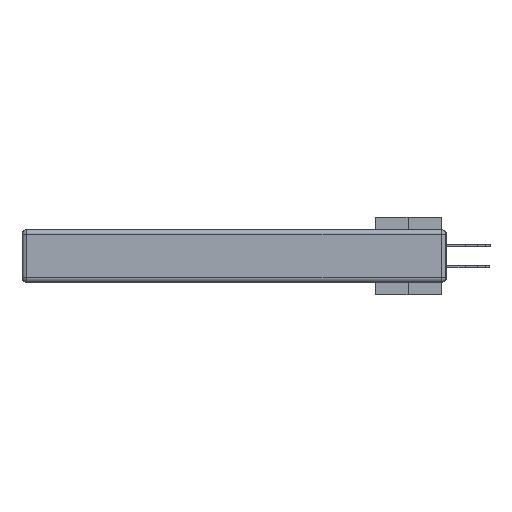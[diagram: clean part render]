
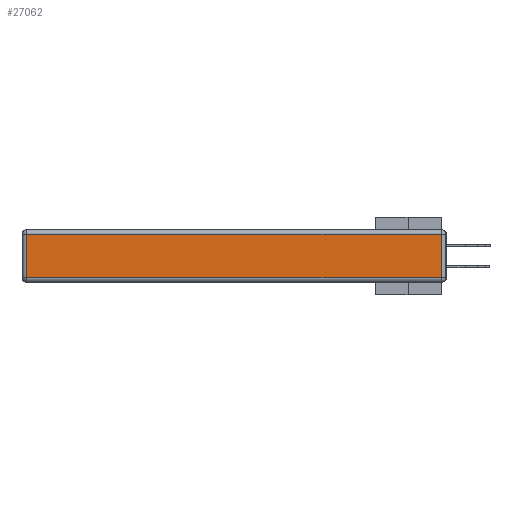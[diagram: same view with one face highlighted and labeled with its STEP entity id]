
A CAD part, left-side view. The second image highlights one B-rep face of the part: STEP entity #27062.
In plain terms, the highlighted planar face has unit normal (-1, 0, 0).
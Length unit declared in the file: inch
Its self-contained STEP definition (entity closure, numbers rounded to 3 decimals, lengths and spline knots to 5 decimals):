
#380 = VERTEX_POINT ( 'NONE', #498 ) ;
#498 = CARTESIAN_POINT ( 'NONE',  ( 0., 0.03, -0.03 ) ) ;
#3220 = VECTOR ( 'NONE', #11821, 39.37008 ) ;
#5016 = CARTESIAN_POINT ( 'NONE',  ( 0., 0., -0.343 ) ) ;
#7217 = VERTEX_POINT ( 'NONE', #21362 ) ;
#7715 = CARTESIAN_POINT ( 'NONE',  ( 0., 0.03, -0.313 ) ) ;
#9782 = VECTOR ( 'NONE', #29040, 39.37008 ) ;
#9840 = ORIENTED_EDGE ( 'NONE', *, *, #22246, .T. ) ;
#11810 = EDGE_CURVE ( 'NONE', #7217, #14208, #23583, .T. ) ;
#11821 = DIRECTION ( 'NONE',  ( 0., 0., 1. ) ) ;
#12468 = EDGE_CURVE ( 'NONE', #20506, #7217, #20412, .T. ) ;
#13033 = CARTESIAN_POINT ( 'NONE',  ( 0., 0., -0.313 ) ) ;
#14208 = VERTEX_POINT ( 'NONE', #7715 ) ;
#14841 = DIRECTION ( 'NONE',  ( 0., 0., 1. ) ) ;
#16550 = LINE ( 'NONE', #27751, #32990 ) ;
#17614 = CARTESIAN_POINT ( 'NONE',  ( 0., 2.72, -0.343 ) ) ;
#17719 = PLANE ( 'NONE',  #21670 ) ;
#17852 = VECTOR ( 'NONE', #21187, 39.37008 ) ;
#18949 = FACE_OUTER_BOUND ( 'NONE', #33417, .T. ) ;
#20294 = ORIENTED_EDGE ( 'NONE', *, *, #11810, .T. ) ;
#20412 = LINE ( 'NONE', #17614, #17852 ) ;
#20506 = VERTEX_POINT ( 'NONE', #30685 ) ;
#21187 = DIRECTION ( 'NONE',  ( 0., 0., -1. ) ) ;
#21362 = CARTESIAN_POINT ( 'NONE',  ( 0., 2.72, -0.313 ) ) ;
#21670 = AXIS2_PLACEMENT_3D ( 'NONE', #5016, #33962, #14841 ) ;
#22246 = EDGE_CURVE ( 'NONE', #14208, #380, #25757, .T. ) ;
#23583 = LINE ( 'NONE', #13033, #9782 ) ;
#25087 = CARTESIAN_POINT ( 'NONE',  ( 0., 0.03, -0.343 ) ) ;
#25757 = LINE ( 'NONE', #25087, #3220 ) ;
#27062 = ADVANCED_FACE ( 'NONE', ( #18949 ), #17719, .T. ) ;
#27751 = CARTESIAN_POINT ( 'NONE',  ( 0., 2.75, -0.03 ) ) ;
#28865 = ORIENTED_EDGE ( 'NONE', *, *, #39782, .T. ) ;
#29040 = DIRECTION ( 'NONE',  ( 0., -1., 0. ) ) ;
#30685 = CARTESIAN_POINT ( 'NONE',  ( 0., 2.72, -0.03 ) ) ;
#32990 = VECTOR ( 'NONE', #34261, 39.37008 ) ;
#33417 = EDGE_LOOP ( 'NONE', ( #20294, #9840, #28865, #37690 ) ) ;
#33962 = DIRECTION ( 'NONE',  ( -1., 0., 0. ) ) ;
#34261 = DIRECTION ( 'NONE',  ( 0., 1., 0. ) ) ;
#37690 = ORIENTED_EDGE ( 'NONE', *, *, #12468, .T. ) ;
#39782 = EDGE_CURVE ( 'NONE', #380, #20506, #16550, .T. ) ;
